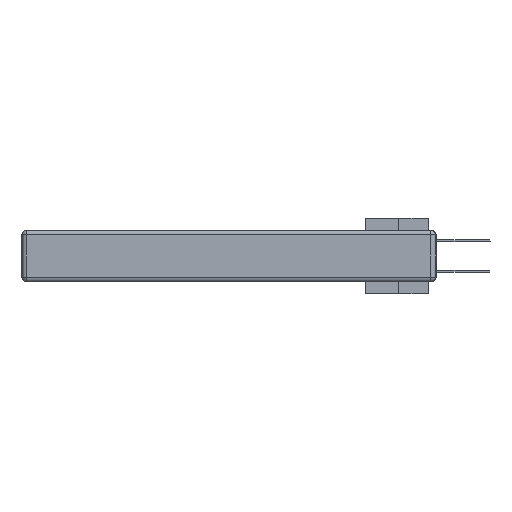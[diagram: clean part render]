
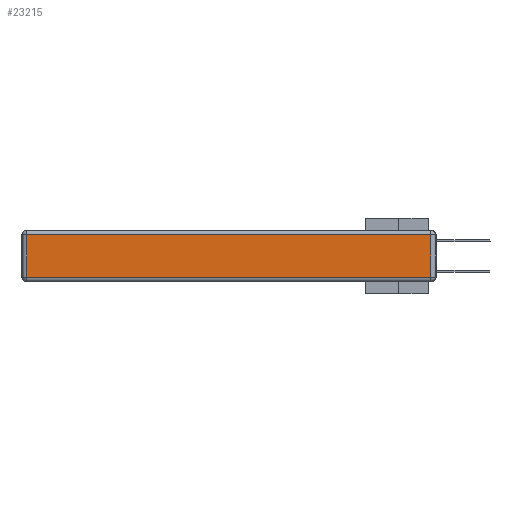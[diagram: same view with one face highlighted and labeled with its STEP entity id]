
A CAD part, left-side view. The second image highlights one B-rep face of the part: STEP entity #23215.
In plain terms, the highlighted planar face has unit normal (-1, 0, 0).
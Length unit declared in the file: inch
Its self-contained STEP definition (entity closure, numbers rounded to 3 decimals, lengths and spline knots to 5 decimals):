
#24 = CARTESIAN_POINT ( 'NONE',  ( 0., 0.03, -0.313 ) ) ;
#743 = VERTEX_POINT ( 'NONE', #24 ) ;
#4336 = FACE_OUTER_BOUND ( 'NONE', #37573, .T. ) ;
#5433 = DIRECTION ( 'NONE',  ( 0., 0., -1. ) ) ;
#6535 = CARTESIAN_POINT ( 'NONE',  ( 0., 0.03, -0.03 ) ) ;
#7118 = DIRECTION ( 'NONE',  ( -1., 0., 0. ) ) ;
#7717 = VERTEX_POINT ( 'NONE', #6535 ) ;
#8206 = LINE ( 'NONE', #8607, #10916 ) ;
#8607 = CARTESIAN_POINT ( 'NONE',  ( 0., 2.72, -0.343 ) ) ;
#8873 = ORIENTED_EDGE ( 'NONE', *, *, #24299, .T. ) ;
#9811 = VERTEX_POINT ( 'NONE', #21890 ) ;
#10899 = ORIENTED_EDGE ( 'NONE', *, *, #32695, .T. ) ;
#10916 = VECTOR ( 'NONE', #5433, 39.37008 ) ;
#11640 = VECTOR ( 'NONE', #35928, 39.37008 ) ;
#12409 = VERTEX_POINT ( 'NONE', #29212 ) ;
#12787 = DIRECTION ( 'NONE',  ( 0., -1., 0. ) ) ;
#16063 = ORIENTED_EDGE ( 'NONE', *, *, #16564, .T. ) ;
#16101 = CARTESIAN_POINT ( 'NONE',  ( 0., 2.75, -0.03 ) ) ;
#16564 = EDGE_CURVE ( 'NONE', #7717, #12409, #28475, .T. ) ;
#17960 = AXIS2_PLACEMENT_3D ( 'NONE', #19029, #7118, #19632 ) ;
#19029 = CARTESIAN_POINT ( 'NONE',  ( 0., 0., -0.343 ) ) ;
#19632 = DIRECTION ( 'NONE',  ( 0., 0., 1. ) ) ;
#21890 = CARTESIAN_POINT ( 'NONE',  ( 0., 2.72, -0.313 ) ) ;
#22217 = ORIENTED_EDGE ( 'NONE', *, *, #32467, .T. ) ;
#23215 = ADVANCED_FACE ( 'NONE', ( #4336 ), #37417, .T. ) ;
#24299 = EDGE_CURVE ( 'NONE', #12409, #9811, #8206, .T. ) ;
#25626 = VECTOR ( 'NONE', #12787, 39.37008 ) ;
#28475 = LINE ( 'NONE', #16101, #29775 ) ;
#29212 = CARTESIAN_POINT ( 'NONE',  ( 0., 2.72, -0.03 ) ) ;
#29702 = CARTESIAN_POINT ( 'NONE',  ( 0., 0.03, -0.343 ) ) ;
#29775 = VECTOR ( 'NONE', #31865, 39.37008 ) ;
#30295 = LINE ( 'NONE', #29702, #11640 ) ;
#31865 = DIRECTION ( 'NONE',  ( 0., 1., 0. ) ) ;
#32467 = EDGE_CURVE ( 'NONE', #9811, #743, #33928, .T. ) ;
#32695 = EDGE_CURVE ( 'NONE', #743, #7717, #30295, .T. ) ;
#33723 = CARTESIAN_POINT ( 'NONE',  ( 0., 0., -0.313 ) ) ;
#33928 = LINE ( 'NONE', #33723, #25626 ) ;
#35928 = DIRECTION ( 'NONE',  ( 0., 0., 1. ) ) ;
#37417 = PLANE ( 'NONE',  #17960 ) ;
#37573 = EDGE_LOOP ( 'NONE', ( #22217, #10899, #16063, #8873 ) ) ;
